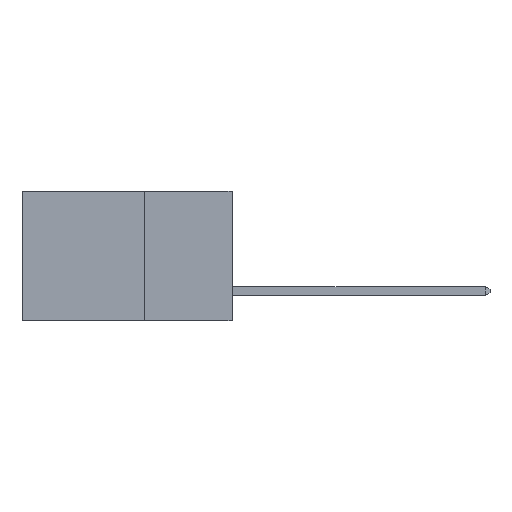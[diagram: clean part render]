
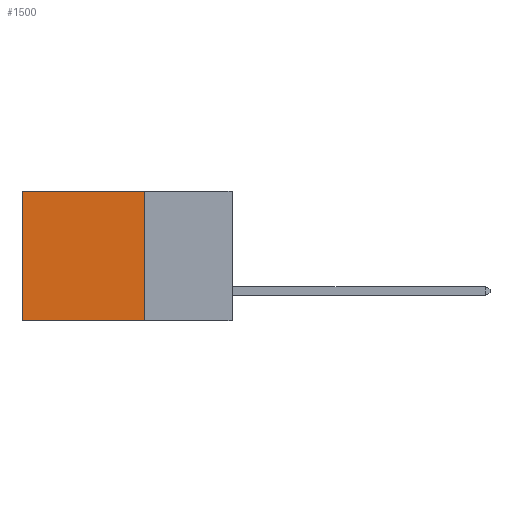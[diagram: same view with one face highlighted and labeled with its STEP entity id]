
A CAD part, left-side view. The second image highlights one B-rep face of the part: STEP entity #1500.
In plain terms, the highlighted planar face has unit normal (-1, 0, 0).
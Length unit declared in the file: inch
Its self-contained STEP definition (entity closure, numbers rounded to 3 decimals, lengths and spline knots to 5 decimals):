
#52 = EDGE_CURVE ( 'NONE', #9924, #12002, #9203, .T. ) ;
#152 = CARTESIAN_POINT ( 'NONE',  ( 0.2875, 0.25, -0.37 ) ) ;
#1500 = ADVANCED_FACE ( 'NONE', ( #18908 ), #17597, .F. ) ;
#1596 = DIRECTION ( 'NONE',  ( 0., 1., 0. ) ) ;
#2197 = DIRECTION ( 'NONE',  ( 0., 1., 0. ) ) ;
#2214 = CARTESIAN_POINT ( 'NONE',  ( 0.2875, 0.25, -0.37 ) ) ;
#2297 = ORIENTED_EDGE ( 'NONE', *, *, #8649, .F. ) ;
#3084 = AXIS2_PLACEMENT_3D ( 'NONE', #13230, #19054, #10391 ) ;
#3105 = VERTEX_POINT ( 'NONE', #14514 ) ;
#3148 = VECTOR ( 'NONE', #1596, 39.37008 ) ;
#5470 = VECTOR ( 'NONE', #2197, 39.37008 ) ;
#6465 = DIRECTION ( 'NONE',  ( 0., 0., -1. ) ) ;
#6856 = LINE ( 'NONE', #18237, #13857 ) ;
#6945 = LINE ( 'NONE', #8109, #3148 ) ;
#7042 = ORIENTED_EDGE ( 'NONE', *, *, #13430, .T. ) ;
#7179 = LINE ( 'NONE', #8584, #14604 ) ;
#8109 = CARTESIAN_POINT ( 'NONE',  ( 0.2875, 0.25, 0. ) ) ;
#8584 = CARTESIAN_POINT ( 'NONE',  ( 0.2875, 0.6, 0. ) ) ;
#8649 = EDGE_CURVE ( 'NONE', #19657, #9924, #6856, .T. ) ;
#8769 = CARTESIAN_POINT ( 'NONE',  ( 0.2875, 0.6, -0.37 ) ) ;
#8871 = ORIENTED_EDGE ( 'NONE', *, *, #12446, .T. ) ;
#9203 = LINE ( 'NONE', #2214, #5470 ) ;
#9381 = EDGE_LOOP ( 'NONE', ( #7042, #10418, #2297, #8871 ) ) ;
#9924 = VERTEX_POINT ( 'NONE', #152 ) ;
#10391 = DIRECTION ( 'NONE',  ( 0., 0., -1. ) ) ;
#10418 = ORIENTED_EDGE ( 'NONE', *, *, #52, .F. ) ;
#12002 = VERTEX_POINT ( 'NONE', #8769 ) ;
#12446 = EDGE_CURVE ( 'NONE', #19657, #3105, #6945, .T. ) ;
#13230 = CARTESIAN_POINT ( 'NONE',  ( 0.2875, 0.25, 0. ) ) ;
#13430 = EDGE_CURVE ( 'NONE', #3105, #12002, #7179, .T. ) ;
#13857 = VECTOR ( 'NONE', #6465, 39.37008 ) ;
#14514 = CARTESIAN_POINT ( 'NONE',  ( 0.2875, 0.6, 0. ) ) ;
#14604 = VECTOR ( 'NONE', #18732, 39.37008 ) ;
#15626 = CARTESIAN_POINT ( 'NONE',  ( 0.2875, 0.25, 0. ) ) ;
#17597 = PLANE ( 'NONE',  #3084 ) ;
#18237 = CARTESIAN_POINT ( 'NONE',  ( 0.2875, 0.25, 0. ) ) ;
#18732 = DIRECTION ( 'NONE',  ( 0., 0., -1. ) ) ;
#18908 = FACE_OUTER_BOUND ( 'NONE', #9381, .T. ) ;
#19054 = DIRECTION ( 'NONE',  ( 1., 0., 0. ) ) ;
#19657 = VERTEX_POINT ( 'NONE', #15626 ) ;
